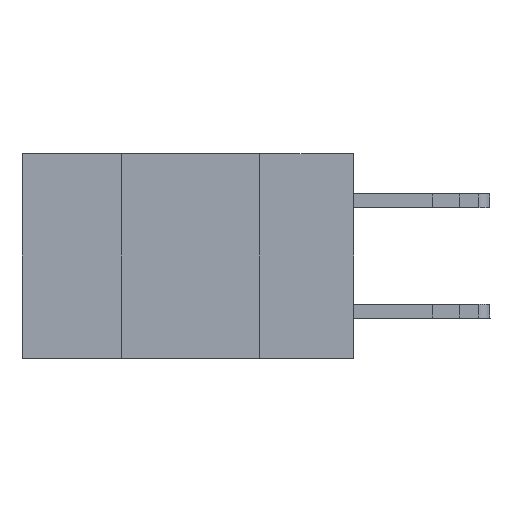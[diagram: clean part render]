
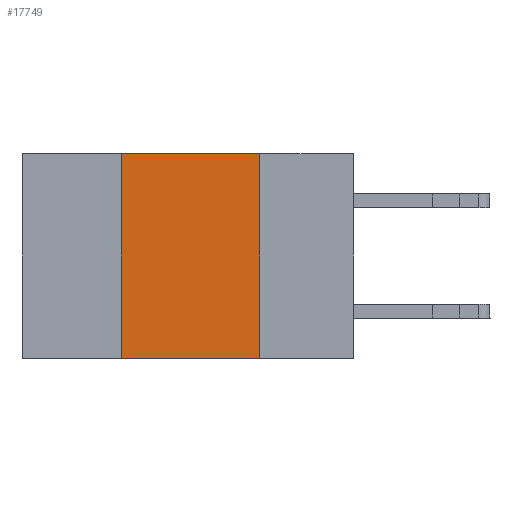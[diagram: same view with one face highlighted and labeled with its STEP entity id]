
A CAD part, left-side view. The second image highlights one B-rep face of the part: STEP entity #17749.
In plain terms, the highlighted planar face has unit normal (-1, 0, 0).
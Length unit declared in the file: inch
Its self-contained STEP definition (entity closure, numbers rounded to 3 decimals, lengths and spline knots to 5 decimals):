
#122 = DIRECTION ( 'NONE',  ( 0., 0., 1. ) ) ;
#688 = CARTESIAN_POINT ( 'NONE',  ( 0., 0.6, 0. ) ) ;
#1193 = DIRECTION ( 'NONE',  ( 0., -1., 0. ) ) ;
#1278 = CARTESIAN_POINT ( 'NONE',  ( 0., 0.6, -0.37 ) ) ;
#1976 = VERTEX_POINT ( 'NONE', #3883 ) ;
#2486 = ORIENTED_EDGE ( 'NONE', *, *, #4229, .F. ) ;
#2613 = DIRECTION ( 'NONE',  ( 0., 0., -1. ) ) ;
#3014 = CARTESIAN_POINT ( 'NONE',  ( 0., 0.42, -0.37 ) ) ;
#3371 = VERTEX_POINT ( 'NONE', #16346 ) ;
#3542 = VERTEX_POINT ( 'NONE', #18220 ) ;
#3818 = AXIS2_PLACEMENT_3D ( 'NONE', #6287, #13332, #2613 ) ;
#3883 = CARTESIAN_POINT ( 'NONE',  ( 0., 0.17, 0. ) ) ;
#4229 = EDGE_CURVE ( 'NONE', #1976, #3542, #14540, .T. ) ;
#5044 = VERTEX_POINT ( 'NONE', #3014 ) ;
#5853 = EDGE_LOOP ( 'NONE', ( #2486, #22426, #18932, #10735 ) ) ;
#6287 = CARTESIAN_POINT ( 'NONE',  ( 0., 0.6, 0. ) ) ;
#7821 = VECTOR ( 'NONE', #122, 39.37008 ) ;
#9293 = VECTOR ( 'NONE', #1193, 39.37008 ) ;
#9888 = VECTOR ( 'NONE', #13038, 39.37008 ) ;
#10735 = ORIENTED_EDGE ( 'NONE', *, *, #11431, .T. ) ;
#11431 = EDGE_CURVE ( 'NONE', #5044, #3542, #18578, .T. ) ;
#11550 = DIRECTION ( 'NONE',  ( 0., -1., 0. ) ) ;
#11606 = PLANE ( 'NONE',  #3818 ) ;
#11975 = LINE ( 'NONE', #688, #16641 ) ;
#13038 = DIRECTION ( 'NONE',  ( 0., 0., -1. ) ) ;
#13332 = DIRECTION ( 'NONE',  ( 1., 0., 0. ) ) ;
#14540 = LINE ( 'NONE', #21768, #9888 ) ;
#15241 = EDGE_CURVE ( 'NONE', #3371, #1976, #11975, .T. ) ;
#16346 = CARTESIAN_POINT ( 'NONE',  ( 0., 0.42, 0. ) ) ;
#16641 = VECTOR ( 'NONE', #11550, 39.37008 ) ;
#16871 = EDGE_CURVE ( 'NONE', #5044, #3371, #17112, .T. ) ;
#17112 = LINE ( 'NONE', #19742, #7821 ) ;
#17749 = ADVANCED_FACE ( 'NONE', ( #21986 ), #11606, .F. ) ;
#18220 = CARTESIAN_POINT ( 'NONE',  ( 0., 0.17, -0.37 ) ) ;
#18578 = LINE ( 'NONE', #1278, #9293 ) ;
#18932 = ORIENTED_EDGE ( 'NONE', *, *, #16871, .F. ) ;
#19742 = CARTESIAN_POINT ( 'NONE',  ( 0., 0.42, 0. ) ) ;
#21768 = CARTESIAN_POINT ( 'NONE',  ( 0., 0.17, 0. ) ) ;
#21986 = FACE_OUTER_BOUND ( 'NONE', #5853, .T. ) ;
#22426 = ORIENTED_EDGE ( 'NONE', *, *, #15241, .F. ) ;
